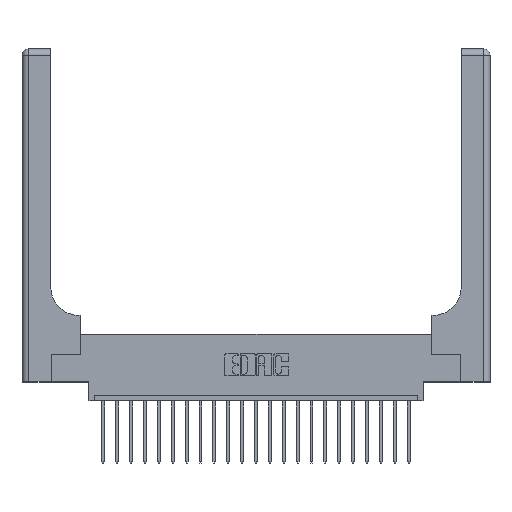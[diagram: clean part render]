
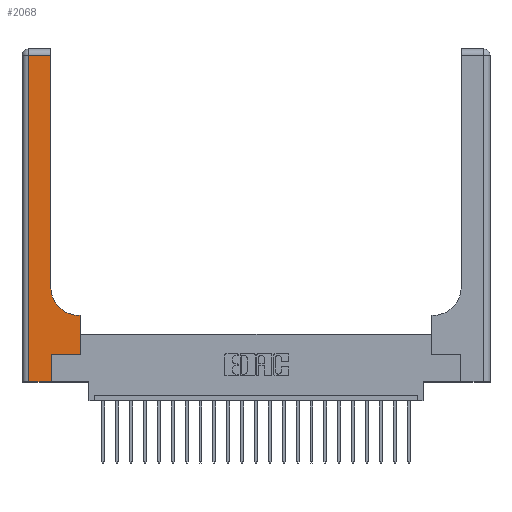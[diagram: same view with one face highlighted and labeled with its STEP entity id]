
A CAD part, top view. The second image highlights one B-rep face of the part: STEP entity #2068.
In plain terms, the highlighted planar face has unit normal (0, 0, 1).
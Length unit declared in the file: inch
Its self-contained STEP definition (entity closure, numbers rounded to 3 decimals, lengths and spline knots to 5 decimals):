
#170 = ORIENTED_EDGE ( 'NONE', *, *, #11290, .T. ) ;
#515 = EDGE_CURVE ( 'NONE', #14177, #1311, #22002, .T. ) ;
#582 = ORIENTED_EDGE ( 'NONE', *, *, #3343, .T. ) ;
#683 = LINE ( 'NONE', #16306, #2993 ) ;
#835 = FACE_OUTER_BOUND ( 'NONE', #3021, .T. ) ;
#983 = DIRECTION ( 'NONE',  ( 1., 0., 0. ) ) ;
#1208 = EDGE_CURVE ( 'NONE', #1311, #15000, #10021, .T. ) ;
#1311 = VERTEX_POINT ( 'NONE', #7238 ) ;
#1748 = ORIENTED_EDGE ( 'NONE', *, *, #8228, .T. ) ;
#2068 = ADVANCED_FACE ( 'NONE', ( #835 ), #6288, .F. ) ;
#2131 = AXIS2_PLACEMENT_3D ( 'NONE', #14753, #8149, #11346 ) ;
#2883 = LINE ( 'NONE', #18388, #2911 ) ;
#2911 = VECTOR ( 'NONE', #15100, 39.37008 ) ;
#2951 = DIRECTION ( 'NONE',  ( 0., 1., 0. ) ) ;
#2993 = VECTOR ( 'NONE', #19961, 39.37008 ) ;
#3021 = EDGE_LOOP ( 'NONE', ( #21695, #582, #5269, #18857, #13136, #3875, #1748, #170, #11492 ) ) ;
#3343 = EDGE_CURVE ( 'NONE', #5376, #9561, #7524, .T. ) ;
#3875 = ORIENTED_EDGE ( 'NONE', *, *, #4979, .T. ) ;
#4324 = CARTESIAN_POINT ( 'NONE',  ( 0.51, 0.85, 0.37 ) ) ;
#4883 = EDGE_CURVE ( 'NONE', #18468, #5376, #5782, .T. ) ;
#4979 = EDGE_CURVE ( 'NONE', #15000, #15540, #683, .T. ) ;
#5260 = CARTESIAN_POINT ( 'NONE',  ( 0.06, 2.94, 0.37 ) ) ;
#5269 = ORIENTED_EDGE ( 'NONE', *, *, #8536, .T. ) ;
#5376 = VERTEX_POINT ( 'NONE', #11269 ) ;
#5782 = LINE ( 'NONE', #21686, #7321 ) ;
#6223 = EDGE_CURVE ( 'NONE', #15965, #18468, #21349, .T. ) ;
#6288 = PLANE ( 'NONE',  #2131 ) ;
#7238 = CARTESIAN_POINT ( 'NONE',  ( 0.265, 0., 0.37 ) ) ;
#7310 = VECTOR ( 'NONE', #9344, 39.37008 ) ;
#7321 = VECTOR ( 'NONE', #9468, 39.37008 ) ;
#7524 = LINE ( 'NONE', #7647, #18225 ) ;
#7563 = VECTOR ( 'NONE', #14331, 39.37008 ) ;
#7647 = CARTESIAN_POINT ( 'NONE',  ( 0., 2.94, 0.37 ) ) ;
#7778 = CARTESIAN_POINT ( 'NONE',  ( 0.265, 0.25, 0.37 ) ) ;
#8149 = DIRECTION ( 'NONE',  ( 0., 0., -1. ) ) ;
#8228 = EDGE_CURVE ( 'NONE', #15540, #18200, #8858, .T. ) ;
#8536 = EDGE_CURVE ( 'NONE', #9561, #14177, #2883, .T. ) ;
#8858 = LINE ( 'NONE', #12330, #7563 ) ;
#9344 = DIRECTION ( 'NONE',  ( -1., 0., 0. ) ) ;
#9468 = DIRECTION ( 'NONE',  ( 0., 1., 0. ) ) ;
#9483 = DIRECTION ( 'NONE',  ( -1., 0., 0. ) ) ;
#9561 = VERTEX_POINT ( 'NONE', #5260 ) ;
#9957 = CARTESIAN_POINT ( 'NONE',  ( 0.26, 0.85, 0.37 ) ) ;
#10021 = LINE ( 'NONE', #13442, #12662 ) ;
#11269 = CARTESIAN_POINT ( 'NONE',  ( 0.26, 2.94, 0.37 ) ) ;
#11290 = EDGE_CURVE ( 'NONE', #18200, #15965, #21239, .T. ) ;
#11310 = DIRECTION ( 'NONE',  ( 0., 0., -1. ) ) ;
#11346 = DIRECTION ( 'NONE',  ( -1., 0., 0. ) ) ;
#11492 = ORIENTED_EDGE ( 'NONE', *, *, #6223, .T. ) ;
#12330 = CARTESIAN_POINT ( 'NONE',  ( 0.528, 0.25, 0.37 ) ) ;
#12662 = VECTOR ( 'NONE', #2951, 39.37008 ) ;
#12810 = CARTESIAN_POINT ( 'NONE',  ( 0.51, 0.6, 0.37 ) ) ;
#13136 = ORIENTED_EDGE ( 'NONE', *, *, #1208, .T. ) ;
#13442 = CARTESIAN_POINT ( 'NONE',  ( 0.265, 0., 0.37 ) ) ;
#14177 = VERTEX_POINT ( 'NONE', #16502 ) ;
#14331 = DIRECTION ( 'NONE',  ( 0., 1., 0. ) ) ;
#14753 = CARTESIAN_POINT ( 'NONE',  ( 0., 3., 0.37 ) ) ;
#15000 = VERTEX_POINT ( 'NONE', #7778 ) ;
#15018 = CARTESIAN_POINT ( 'NONE',  ( 0., 0., 0.37 ) ) ;
#15077 = DIRECTION ( 'NONE',  ( 1., 0., 0. ) ) ;
#15100 = DIRECTION ( 'NONE',  ( 0., -1., 0. ) ) ;
#15540 = VERTEX_POINT ( 'NONE', #19021 ) ;
#15965 = VERTEX_POINT ( 'NONE', #12810 ) ;
#16306 = CARTESIAN_POINT ( 'NONE',  ( 0.265, 0.25, 0.37 ) ) ;
#16502 = CARTESIAN_POINT ( 'NONE',  ( 0.06, 0., 0.37 ) ) ;
#18200 = VERTEX_POINT ( 'NONE', #21152 ) ;
#18225 = VECTOR ( 'NONE', #9483, 39.37008 ) ;
#18388 = CARTESIAN_POINT ( 'NONE',  ( 0.06, 3., 0.37 ) ) ;
#18468 = VERTEX_POINT ( 'NONE', #9957 ) ;
#18796 = AXIS2_PLACEMENT_3D ( 'NONE', #4324, #11310, #15077 ) ;
#18857 = ORIENTED_EDGE ( 'NONE', *, *, #515, .T. ) ;
#19021 = CARTESIAN_POINT ( 'NONE',  ( 0.528, 0.25, 0.37 ) ) ;
#19725 = CARTESIAN_POINT ( 'NONE',  ( 0.26, 0.6, 0.37 ) ) ;
#19961 = DIRECTION ( 'NONE',  ( 1., 0., 0. ) ) ;
#21152 = CARTESIAN_POINT ( 'NONE',  ( 0.528, 0.6, 0.37 ) ) ;
#21239 = LINE ( 'NONE', #19725, #7310 ) ;
#21349 = CIRCLE ( 'NONE', #18796, 0.25 ) ;
#21686 = CARTESIAN_POINT ( 'NONE',  ( 0.26, 3., 0.37 ) ) ;
#21695 = ORIENTED_EDGE ( 'NONE', *, *, #4883, .T. ) ;
#22002 = LINE ( 'NONE', #15018, #22121 ) ;
#22121 = VECTOR ( 'NONE', #983, 39.37008 ) ;
